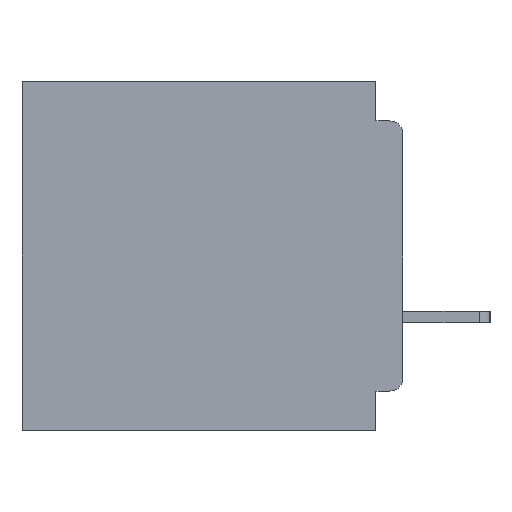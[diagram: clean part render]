
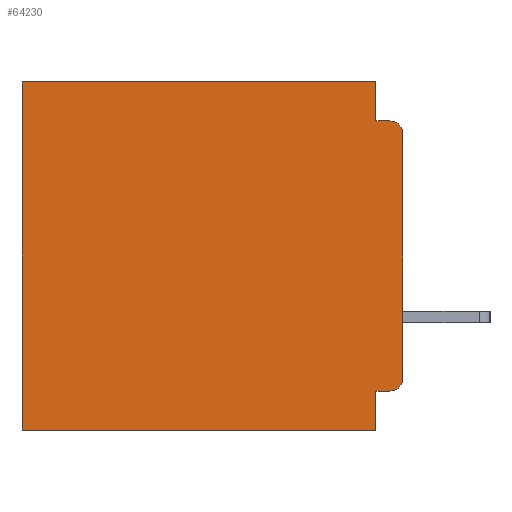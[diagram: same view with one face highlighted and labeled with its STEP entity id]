
A CAD part, left-side view. The second image highlights one B-rep face of the part: STEP entity #64230.
In plain terms, the highlighted planar face has unit normal (-1, 0, 0).
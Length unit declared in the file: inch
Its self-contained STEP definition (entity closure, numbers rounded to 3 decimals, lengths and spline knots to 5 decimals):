
#328 = DIRECTION ( 'NONE',  ( 0., 1., 0. ) ) ;
#896 = DIRECTION ( 'NONE',  ( 0., -1., 0. ) ) ;
#1302 = LINE ( 'NONE', #13495, #53949 ) ;
#2029 = ORIENTED_EDGE ( 'NONE', *, *, #22572, .F. ) ;
#2044 = ORIENTED_EDGE ( 'NONE', *, *, #45106, .T. ) ;
#2314 = VERTEX_POINT ( 'NONE', #5480 ) ;
#3103 = CARTESIAN_POINT ( 'NONE',  ( 0.3, 0., -0.06 ) ) ;
#3370 = ORIENTED_EDGE ( 'NONE', *, *, #11847, .F. ) ;
#4033 = EDGE_CURVE ( 'NONE', #2314, #57568, #22924, .T. ) ;
#4036 = CIRCLE ( 'NONE', #54631, 0.015 ) ;
#5064 = DIRECTION ( 'NONE',  ( 0., 1., 0. ) ) ;
#5258 = LINE ( 'NONE', #30240, #53065 ) ;
#5480 = CARTESIAN_POINT ( 'NONE',  ( 0.3, 0.031, 0. ) ) ;
#7102 = VECTOR ( 'NONE', #5064, 39.37008 ) ;
#7567 = DIRECTION ( 'NONE',  ( 0., 0., -1. ) ) ;
#8412 = CARTESIAN_POINT ( 'NONE',  ( 0.3, 0.437, -0.4 ) ) ;
#9362 = VECTOR ( 'NONE', #10615, 39.37008 ) ;
#10615 = DIRECTION ( 'NONE',  ( 0., 1., 0. ) ) ;
#10913 = EDGE_CURVE ( 'NONE', #2314, #27334, #58941, .T. ) ;
#11847 = EDGE_CURVE ( 'NONE', #42565, #59280, #5258, .T. ) ;
#12008 = EDGE_CURVE ( 'NONE', #27334, #25864, #41938, .T. ) ;
#13011 = DIRECTION ( 'NONE',  ( 1., 0., 0. ) ) ;
#13495 = CARTESIAN_POINT ( 'NONE',  ( 0.3, 0.031, -0.4 ) ) ;
#14692 = ORIENTED_EDGE ( 'NONE', *, *, #23498, .F. ) ;
#14867 = VECTOR ( 'NONE', #896, 39.37008 ) ;
#14934 = EDGE_CURVE ( 'NONE', #57568, #33465, #18510, .T. ) ;
#15984 = ORIENTED_EDGE ( 'NONE', *, *, #14934, .T. ) ;
#18510 = LINE ( 'NONE', #38186, #27222 ) ;
#19089 = CARTESIAN_POINT ( 'NONE',  ( 0.3, 0., 0. ) ) ;
#22092 = CIRCLE ( 'NONE', #27255, 0.015 ) ;
#22531 = DIRECTION ( 'NONE',  ( -1., 0., 0. ) ) ;
#22572 = EDGE_CURVE ( 'NONE', #63210, #42678, #1302, .T. ) ;
#22924 = LINE ( 'NONE', #19089, #9362 ) ;
#23498 = EDGE_CURVE ( 'NONE', #24245, #63210, #42763, .T. ) ;
#23920 = FACE_OUTER_BOUND ( 'NONE', #40223, .T. ) ;
#24245 = VERTEX_POINT ( 'NONE', #57688 ) ;
#24373 = CARTESIAN_POINT ( 'NONE',  ( 0.3, 0.031, -0.4 ) ) ;
#25015 = CARTESIAN_POINT ( 'NONE',  ( 0.3, 0.031, -0.355 ) ) ;
#25864 = VERTEX_POINT ( 'NONE', #38313 ) ;
#26044 = CARTESIAN_POINT ( 'NONE',  ( 0.3, 0., -0.355 ) ) ;
#27222 = VECTOR ( 'NONE', #38391, 39.37008 ) ;
#27255 = AXIS2_PLACEMENT_3D ( 'NONE', #53013, #22531, #58044 ) ;
#27334 = VERTEX_POINT ( 'NONE', #29663 ) ;
#28630 = DIRECTION ( 'NONE',  ( -1., 0., 0. ) ) ;
#29663 = CARTESIAN_POINT ( 'NONE',  ( 0.3, 0.031, -0.045 ) ) ;
#30240 = CARTESIAN_POINT ( 'NONE',  ( 0.3, 0., -0.4 ) ) ;
#32498 = ORIENTED_EDGE ( 'NONE', *, *, #12008, .F. ) ;
#32998 = CARTESIAN_POINT ( 'NONE',  ( 0.3, 0.031, 0. ) ) ;
#33141 = AXIS2_PLACEMENT_3D ( 'NONE', #53690, #13011, #63750 ) ;
#33465 = VERTEX_POINT ( 'NONE', #8412 ) ;
#33848 = ORIENTED_EDGE ( 'NONE', *, *, #37910, .T. ) ;
#35151 = DIRECTION ( 'NONE',  ( 0., 0., -1. ) ) ;
#36690 = CARTESIAN_POINT ( 'NONE',  ( 0.3, 0., -0.045 ) ) ;
#37910 = EDGE_CURVE ( 'NONE', #42565, #25864, #4036, .T. ) ;
#38186 = CARTESIAN_POINT ( 'NONE',  ( 0.3, 0.437, -0.4 ) ) ;
#38313 = CARTESIAN_POINT ( 'NONE',  ( 0.3, 0.015, -0.045 ) ) ;
#38391 = DIRECTION ( 'NONE',  ( 0., 0., -1. ) ) ;
#40223 = EDGE_LOOP ( 'NONE', ( #3370, #33848, #32498, #47454, #44442, #15984, #56485, #2029, #14692, #2044 ) ) ;
#40650 = LINE ( 'NONE', #56064, #7102 ) ;
#41938 = LINE ( 'NONE', #36690, #14867 ) ;
#42565 = VERTEX_POINT ( 'NONE', #3103 ) ;
#42678 = VERTEX_POINT ( 'NONE', #24373 ) ;
#42763 = LINE ( 'NONE', #26044, #53067 ) ;
#44442 = ORIENTED_EDGE ( 'NONE', *, *, #4033, .T. ) ;
#45106 = EDGE_CURVE ( 'NONE', #24245, #59280, #22092, .T. ) ;
#45538 = VECTOR ( 'NONE', #7567, 39.37008 ) ;
#45702 = CARTESIAN_POINT ( 'NONE',  ( 0.3, 0., -0.34 ) ) ;
#47454 = ORIENTED_EDGE ( 'NONE', *, *, #10913, .F. ) ;
#47880 = EDGE_CURVE ( 'NONE', #42678, #33465, #40650, .T. ) ;
#52336 = CARTESIAN_POINT ( 'NONE',  ( 0.3, 0.437, 0. ) ) ;
#53013 = CARTESIAN_POINT ( 'NONE',  ( 0.3, 0.015, -0.34 ) ) ;
#53065 = VECTOR ( 'NONE', #35151, 39.37008 ) ;
#53067 = VECTOR ( 'NONE', #328, 39.37008 ) ;
#53690 = CARTESIAN_POINT ( 'NONE',  ( 0.3, 0., -0.4 ) ) ;
#53949 = VECTOR ( 'NONE', #59217, 39.37008 ) ;
#54631 = AXIS2_PLACEMENT_3D ( 'NONE', #59028, #28630, #64050 ) ;
#56064 = CARTESIAN_POINT ( 'NONE',  ( 0.3, 0., -0.4 ) ) ;
#56485 = ORIENTED_EDGE ( 'NONE', *, *, #47880, .F. ) ;
#57568 = VERTEX_POINT ( 'NONE', #52336 ) ;
#57688 = CARTESIAN_POINT ( 'NONE',  ( 0.3, 0.015, -0.355 ) ) ;
#58044 = DIRECTION ( 'NONE',  ( 0., 0., -1. ) ) ;
#58743 = PLANE ( 'NONE',  #33141 ) ;
#58941 = LINE ( 'NONE', #32998, #45538 ) ;
#59028 = CARTESIAN_POINT ( 'NONE',  ( 0.3, 0.015, -0.06 ) ) ;
#59217 = DIRECTION ( 'NONE',  ( 0., 0., -1. ) ) ;
#59280 = VERTEX_POINT ( 'NONE', #45702 ) ;
#63210 = VERTEX_POINT ( 'NONE', #25015 ) ;
#63750 = DIRECTION ( 'NONE',  ( 0., 0., -1. ) ) ;
#64050 = DIRECTION ( 'NONE',  ( 0., 0., -1. ) ) ;
#64230 = ADVANCED_FACE ( 'NONE', ( #23920 ), #58743, .F. ) ;
